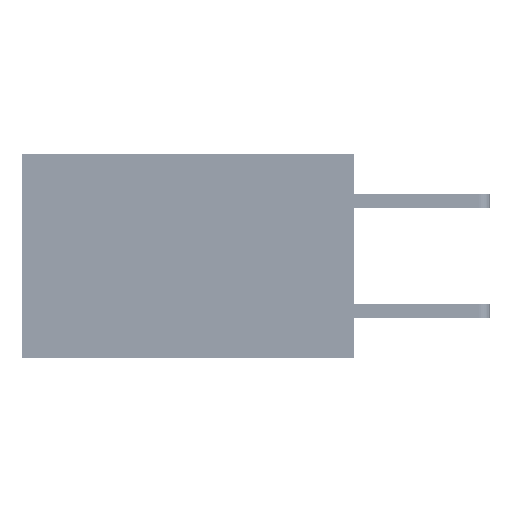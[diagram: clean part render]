
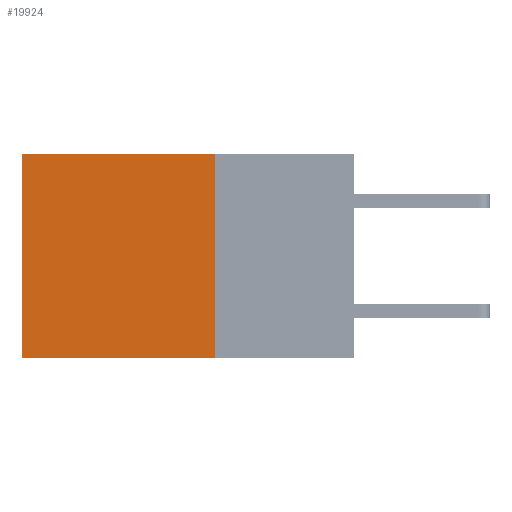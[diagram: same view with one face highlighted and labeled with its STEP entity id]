
A CAD part, left-side view. The second image highlights one B-rep face of the part: STEP entity #19924.
In plain terms, the highlighted planar face has unit normal (-1, 0, 0).
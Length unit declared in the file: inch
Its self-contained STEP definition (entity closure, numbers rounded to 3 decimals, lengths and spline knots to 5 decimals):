
#426 = CARTESIAN_POINT ( 'NONE',  ( 0.2875, 0.6, 0. ) ) ;
#1131 = CARTESIAN_POINT ( 'NONE',  ( 0.2875, 0.25, -0.37 ) ) ;
#3520 = EDGE_LOOP ( 'NONE', ( #13793, #30420, #26860, #40241 ) ) ;
#4166 = VECTOR ( 'NONE', #13439, 39.37008 ) ;
#5128 = DIRECTION ( 'NONE',  ( 0., 0., -1. ) ) ;
#7002 = CARTESIAN_POINT ( 'NONE',  ( 0.2875, 0.25, 0. ) ) ;
#7444 = VECTOR ( 'NONE', #28529, 39.37008 ) ;
#9355 = LINE ( 'NONE', #39037, #32466 ) ;
#10616 = CARTESIAN_POINT ( 'NONE',  ( 0.2875, 0.6, 0. ) ) ;
#12044 = VERTEX_POINT ( 'NONE', #12982 ) ;
#12982 = CARTESIAN_POINT ( 'NONE',  ( 0.2875, 0.6, -0.37 ) ) ;
#13439 = DIRECTION ( 'NONE',  ( 0., 1., 0. ) ) ;
#13793 = ORIENTED_EDGE ( 'NONE', *, *, #21243, .T. ) ;
#14149 = EDGE_CURVE ( 'NONE', #24149, #12044, #19846, .T. ) ;
#16094 = DIRECTION ( 'NONE',  ( 0., 0., -1. ) ) ;
#19397 = CARTESIAN_POINT ( 'NONE',  ( 0.2875, 0.25, 0. ) ) ;
#19846 = LINE ( 'NONE', #1131, #4166 ) ;
#19924 = ADVANCED_FACE ( 'NONE', ( #25526 ), #22678, .F. ) ;
#20278 = VERTEX_POINT ( 'NONE', #36958 ) ;
#20476 = DIRECTION ( 'NONE',  ( 0., 0., -1. ) ) ;
#21243 = EDGE_CURVE ( 'NONE', #21954, #12044, #30363, .T. ) ;
#21954 = VERTEX_POINT ( 'NONE', #426 ) ;
#22529 = DIRECTION ( 'NONE',  ( 1., 0., 0. ) ) ;
#22678 = PLANE ( 'NONE',  #36205 ) ;
#24137 = LINE ( 'NONE', #7002, #7444 ) ;
#24149 = VERTEX_POINT ( 'NONE', #28464 ) ;
#25526 = FACE_OUTER_BOUND ( 'NONE', #3520, .T. ) ;
#25918 = VECTOR ( 'NONE', #20476, 39.37008 ) ;
#26860 = ORIENTED_EDGE ( 'NONE', *, *, #29404, .F. ) ;
#28464 = CARTESIAN_POINT ( 'NONE',  ( 0.2875, 0.25, -0.37 ) ) ;
#28529 = DIRECTION ( 'NONE',  ( 0., 1., 0. ) ) ;
#29404 = EDGE_CURVE ( 'NONE', #20278, #24149, #9355, .T. ) ;
#30363 = LINE ( 'NONE', #10616, #25918 ) ;
#30420 = ORIENTED_EDGE ( 'NONE', *, *, #14149, .F. ) ;
#32466 = VECTOR ( 'NONE', #5128, 39.37008 ) ;
#36205 = AXIS2_PLACEMENT_3D ( 'NONE', #19397, #22529, #16094 ) ;
#36589 = EDGE_CURVE ( 'NONE', #20278, #21954, #24137, .T. ) ;
#36958 = CARTESIAN_POINT ( 'NONE',  ( 0.2875, 0.25, 0. ) ) ;
#39037 = CARTESIAN_POINT ( 'NONE',  ( 0.2875, 0.25, 0. ) ) ;
#40241 = ORIENTED_EDGE ( 'NONE', *, *, #36589, .T. ) ;
